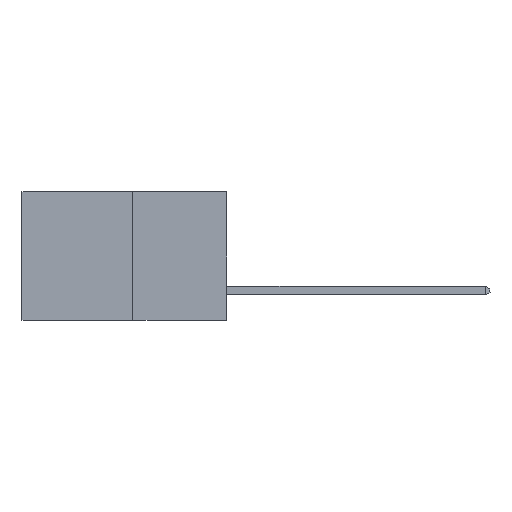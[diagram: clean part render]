
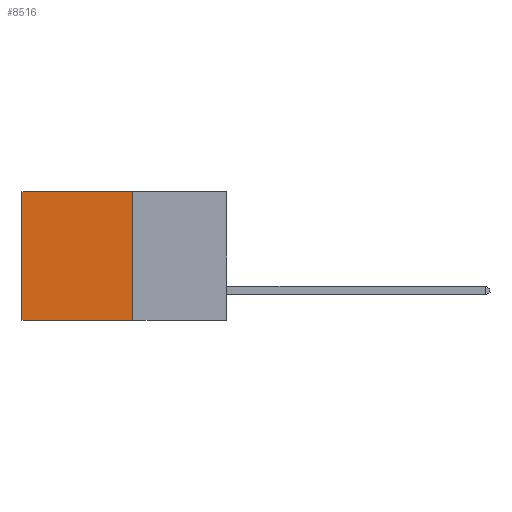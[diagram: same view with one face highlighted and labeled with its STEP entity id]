
A CAD part, left-side view. The second image highlights one B-rep face of the part: STEP entity #8516.
In plain terms, the highlighted planar face has unit normal (-1, 0, 0).
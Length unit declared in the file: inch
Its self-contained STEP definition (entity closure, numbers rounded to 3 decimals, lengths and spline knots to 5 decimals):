
#392 = ORIENTED_EDGE ( 'NONE', *, *, #5335, .F. ) ;
#677 = LINE ( 'NONE', #5562, #2844 ) ;
#772 = VECTOR ( 'NONE', #4346, 39.37008 ) ;
#1510 = VECTOR ( 'NONE', #8851, 39.37008 ) ;
#2556 = CARTESIAN_POINT ( 'NONE',  ( 0.277, 0.59, -0.37 ) ) ;
#2805 = DIRECTION ( 'NONE',  ( 0., 1., 0. ) ) ;
#2844 = VECTOR ( 'NONE', #7024, 39.37008 ) ;
#3227 = LINE ( 'NONE', #4675, #772 ) ;
#4026 = PLANE ( 'NONE',  #8883 ) ;
#4346 = DIRECTION ( 'NONE',  ( 0., 0., -1. ) ) ;
#4379 = DIRECTION ( 'NONE',  ( 0., 0., -1. ) ) ;
#4588 = DIRECTION ( 'NONE',  ( 1., 0., 0. ) ) ;
#4675 = CARTESIAN_POINT ( 'NONE',  ( 0.277, 0.27, -0.37 ) ) ;
#4892 = CARTESIAN_POINT ( 'NONE',  ( 0.277, 0.27, -0.37 ) ) ;
#5163 = EDGE_CURVE ( 'NONE', #6886, #8788, #10451, .T. ) ;
#5335 = EDGE_CURVE ( 'NONE', #7296, #11417, #677, .T. ) ;
#5562 = CARTESIAN_POINT ( 'NONE',  ( 0.277, 0.27, -0.37 ) ) ;
#5766 = VECTOR ( 'NONE', #2805, 39.37008 ) ;
#6886 = VERTEX_POINT ( 'NONE', #6939 ) ;
#6939 = CARTESIAN_POINT ( 'NONE',  ( 0.277, 0.27, 0. ) ) ;
#7024 = DIRECTION ( 'NONE',  ( 0., 1., 0. ) ) ;
#7296 = VERTEX_POINT ( 'NONE', #10734 ) ;
#7300 = FACE_OUTER_BOUND ( 'NONE', #9200, .T. ) ;
#7869 = CARTESIAN_POINT ( 'NONE',  ( 0.277, 0.27, 0. ) ) ;
#7960 = EDGE_CURVE ( 'NONE', #6886, #7296, #3227, .T. ) ;
#8183 = LINE ( 'NONE', #2556, #1510 ) ;
#8516 = ADVANCED_FACE ( 'NONE', ( #7300 ), #4026, .F. ) ;
#8788 = VERTEX_POINT ( 'NONE', #9296 ) ;
#8817 = ORIENTED_EDGE ( 'NONE', *, *, #10250, .T. ) ;
#8851 = DIRECTION ( 'NONE',  ( 0., 0., -1. ) ) ;
#8883 = AXIS2_PLACEMENT_3D ( 'NONE', #4892, #4588, #4379 ) ;
#9200 = EDGE_LOOP ( 'NONE', ( #8817, #392, #11162, #11164 ) ) ;
#9296 = CARTESIAN_POINT ( 'NONE',  ( 0.277, 0.59, 0. ) ) ;
#9413 = CARTESIAN_POINT ( 'NONE',  ( 0.277, 0.59, -0.37 ) ) ;
#10250 = EDGE_CURVE ( 'NONE', #8788, #11417, #8183, .T. ) ;
#10451 = LINE ( 'NONE', #7869, #5766 ) ;
#10734 = CARTESIAN_POINT ( 'NONE',  ( 0.277, 0.27, -0.37 ) ) ;
#11162 = ORIENTED_EDGE ( 'NONE', *, *, #7960, .F. ) ;
#11164 = ORIENTED_EDGE ( 'NONE', *, *, #5163, .T. ) ;
#11417 = VERTEX_POINT ( 'NONE', #9413 ) ;
